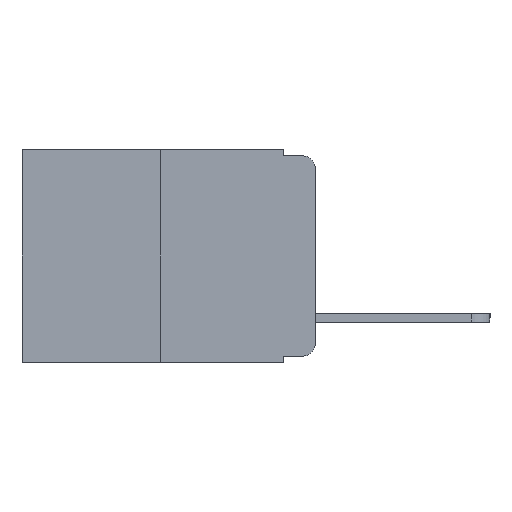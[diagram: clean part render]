
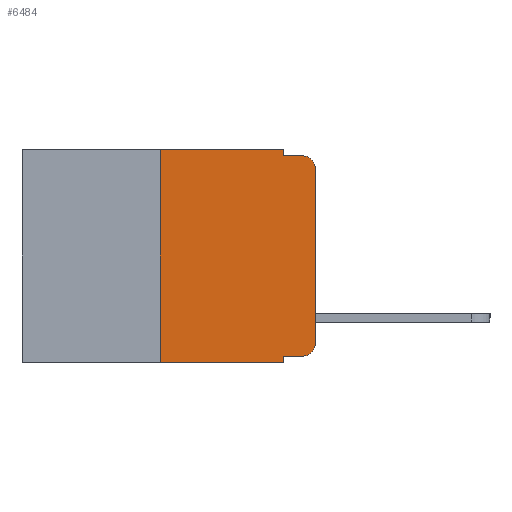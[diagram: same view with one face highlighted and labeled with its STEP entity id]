
A CAD part, left-side view. The second image highlights one B-rep face of the part: STEP entity #6484.
In plain terms, the highlighted planar face has unit normal (-1, 0, 0).
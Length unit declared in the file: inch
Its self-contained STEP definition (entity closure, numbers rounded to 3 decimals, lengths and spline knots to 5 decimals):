
#121 = DIRECTION ( 'NONE',  ( 0., 0., -1. ) ) ;
#460 = ORIENTED_EDGE ( 'NONE', *, *, #2404, .T. ) ;
#630 = ORIENTED_EDGE ( 'NONE', *, *, #4798, .T. ) ;
#737 = DIRECTION ( 'NONE',  ( 0., 0., -1. ) ) ;
#860 = ORIENTED_EDGE ( 'NONE', *, *, #1958, .F. ) ;
#1695 = VECTOR ( 'NONE', #11706, 39.37008 ) ;
#1958 = EDGE_CURVE ( 'NONE', #18882, #8712, #13162, .T. ) ;
#2045 = CARTESIAN_POINT ( 'NONE',  ( 0., 0.051, -0.01 ) ) ;
#2085 = CARTESIAN_POINT ( 'NONE',  ( 0., 0.02, -0.01 ) ) ;
#2247 = LINE ( 'NONE', #12994, #6445 ) ;
#2268 = LINE ( 'NONE', #10017, #1695 ) ;
#2404 = EDGE_CURVE ( 'NONE', #11371, #16719, #4605, .T. ) ;
#2924 = CARTESIAN_POINT ( 'NONE',  ( 0., 0.051, -0.01 ) ) ;
#3169 = EDGE_CURVE ( 'NONE', #14281, #8712, #17897, .T. ) ;
#3745 = AXIS2_PLACEMENT_3D ( 'NONE', #7607, #19991, #9404 ) ;
#4349 = EDGE_CURVE ( 'NONE', #16719, #14281, #2268, .T. ) ;
#4400 = CARTESIAN_POINT ( 'NONE',  ( 0., 0.473, 0. ) ) ;
#4605 = CIRCLE ( 'NONE', #20488, 0.02 ) ;
#4798 = EDGE_CURVE ( 'NONE', #7756, #11371, #2247, .T. ) ;
#4812 = VERTEX_POINT ( 'NONE', #20132 ) ;
#5748 = LINE ( 'NONE', #9719, #14600 ) ;
#6445 = VECTOR ( 'NONE', #14785, 39.37008 ) ;
#6484 = ADVANCED_FACE ( 'NONE', ( #18321 ), #7609, .F. ) ;
#6597 = VECTOR ( 'NONE', #737, 39.37008 ) ;
#6654 = VECTOR ( 'NONE', #7887, 39.37008 ) ;
#6808 = EDGE_LOOP ( 'NONE', ( #15682, #16141, #860, #13383, #13031, #14815, #13010, #14236, #630, #460 ) ) ;
#7426 = DIRECTION ( 'NONE',  ( 0., -1., 0. ) ) ;
#7607 = CARTESIAN_POINT ( 'NONE',  ( 0., 0.02, -0.03 ) ) ;
#7609 = PLANE ( 'NONE',  #9464 ) ;
#7756 = VERTEX_POINT ( 'NONE', #9751 ) ;
#7887 = DIRECTION ( 'NONE',  ( 0., -1., 0. ) ) ;
#8000 = VECTOR ( 'NONE', #17073, 39.37008 ) ;
#8061 = CARTESIAN_POINT ( 'NONE',  ( 0., 0.02, -0.333 ) ) ;
#8369 = EDGE_CURVE ( 'NONE', #7756, #20863, #19589, .T. ) ;
#8481 = VECTOR ( 'NONE', #7426, 39.37008 ) ;
#8712 = VERTEX_POINT ( 'NONE', #2085 ) ;
#9404 = DIRECTION ( 'NONE',  ( 0., 0., -1. ) ) ;
#9464 = AXIS2_PLACEMENT_3D ( 'NONE', #19997, #21753, #11155 ) ;
#9719 = CARTESIAN_POINT ( 'NONE',  ( 0., 0.051, 0. ) ) ;
#9751 = CARTESIAN_POINT ( 'NONE',  ( 0., 0.051, -0.333 ) ) ;
#10017 = CARTESIAN_POINT ( 'NONE',  ( 0., 0., 0. ) ) ;
#10799 = DIRECTION ( 'NONE',  ( -1., 0., 0. ) ) ;
#11155 = DIRECTION ( 'NONE',  ( 0., 0., -1. ) ) ;
#11327 = VECTOR ( 'NONE', #19343, 39.37008 ) ;
#11371 = VERTEX_POINT ( 'NONE', #8061 ) ;
#11706 = DIRECTION ( 'NONE',  ( 0., 0., 1. ) ) ;
#11759 = CARTESIAN_POINT ( 'NONE',  ( 0., 0.473, -0.343 ) ) ;
#12556 = CARTESIAN_POINT ( 'NONE',  ( 0., 0.25, 0. ) ) ;
#12808 = CARTESIAN_POINT ( 'NONE',  ( 0., 0., -0.313 ) ) ;
#12994 = CARTESIAN_POINT ( 'NONE',  ( 0., 0.051, -0.333 ) ) ;
#13010 = ORIENTED_EDGE ( 'NONE', *, *, #15686, .T. ) ;
#13031 = ORIENTED_EDGE ( 'NONE', *, *, #16248, .F. ) ;
#13160 = CARTESIAN_POINT ( 'NONE',  ( 0., 0.051, 0. ) ) ;
#13162 = LINE ( 'NONE', #2045, #8481 ) ;
#13383 = ORIENTED_EDGE ( 'NONE', *, *, #20226, .F. ) ;
#13594 = VERTEX_POINT ( 'NONE', #20218 ) ;
#14236 = ORIENTED_EDGE ( 'NONE', *, *, #8369, .F. ) ;
#14281 = VERTEX_POINT ( 'NONE', #16818 ) ;
#14600 = VECTOR ( 'NONE', #22051, 39.37008 ) ;
#14785 = DIRECTION ( 'NONE',  ( 0., -1., 0. ) ) ;
#14815 = ORIENTED_EDGE ( 'NONE', *, *, #19050, .F. ) ;
#15682 = ORIENTED_EDGE ( 'NONE', *, *, #4349, .T. ) ;
#15686 = EDGE_CURVE ( 'NONE', #4812, #20863, #22097, .T. ) ;
#16141 = ORIENTED_EDGE ( 'NONE', *, *, #3169, .T. ) ;
#16248 = EDGE_CURVE ( 'NONE', #21781, #13594, #20743, .T. ) ;
#16719 = VERTEX_POINT ( 'NONE', #12808 ) ;
#16818 = CARTESIAN_POINT ( 'NONE',  ( 0., 0., -0.03 ) ) ;
#17073 = DIRECTION ( 'NONE',  ( 0., -1., 0. ) ) ;
#17592 = CARTESIAN_POINT ( 'NONE',  ( 0., 0.25, 0. ) ) ;
#17897 = CIRCLE ( 'NONE', #3745, 0.02 ) ;
#18321 = FACE_OUTER_BOUND ( 'NONE', #6808, .T. ) ;
#18882 = VERTEX_POINT ( 'NONE', #2924 ) ;
#19050 = EDGE_CURVE ( 'NONE', #4812, #21781, #21310, .T. ) ;
#19343 = DIRECTION ( 'NONE',  ( 0., 0., 1. ) ) ;
#19589 = LINE ( 'NONE', #13160, #6597 ) ;
#19991 = DIRECTION ( 'NONE',  ( -1., 0., 0. ) ) ;
#19997 = CARTESIAN_POINT ( 'NONE',  ( 0., 0.473, 0. ) ) ;
#20132 = CARTESIAN_POINT ( 'NONE',  ( 0., 0.25, -0.343 ) ) ;
#20218 = CARTESIAN_POINT ( 'NONE',  ( 0., 0.051, 0. ) ) ;
#20226 = EDGE_CURVE ( 'NONE', #13594, #18882, #5748, .T. ) ;
#20488 = AXIS2_PLACEMENT_3D ( 'NONE', #21414, #10799, #121 ) ;
#20743 = LINE ( 'NONE', #4400, #6654 ) ;
#20863 = VERTEX_POINT ( 'NONE', #22415 ) ;
#21310 = LINE ( 'NONE', #17592, #11327 ) ;
#21414 = CARTESIAN_POINT ( 'NONE',  ( 0., 0.02, -0.313 ) ) ;
#21753 = DIRECTION ( 'NONE',  ( 1., 0., 0. ) ) ;
#21781 = VERTEX_POINT ( 'NONE', #12556 ) ;
#22051 = DIRECTION ( 'NONE',  ( 0., 0., -1. ) ) ;
#22097 = LINE ( 'NONE', #11759, #8000 ) ;
#22415 = CARTESIAN_POINT ( 'NONE',  ( 0., 0.051, -0.343 ) ) ;
